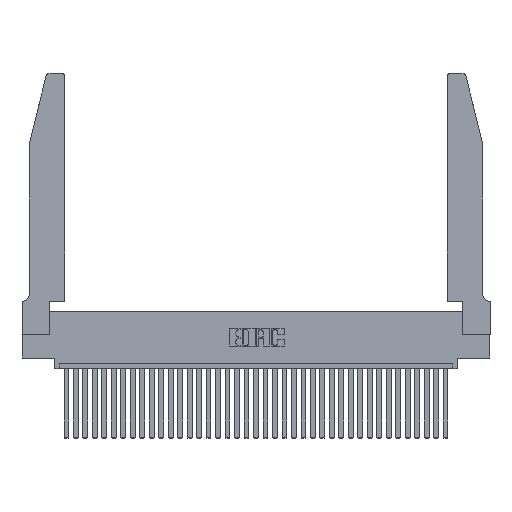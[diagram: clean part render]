
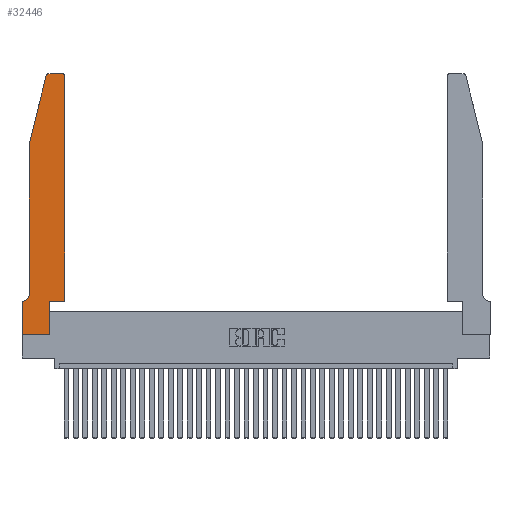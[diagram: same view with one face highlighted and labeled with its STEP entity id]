
A CAD part, top view. The second image highlights one B-rep face of the part: STEP entity #32446.
In plain terms, the highlighted planar face has unit normal (0, 0, 1).
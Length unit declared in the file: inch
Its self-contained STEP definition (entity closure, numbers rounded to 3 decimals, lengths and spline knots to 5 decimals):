
#397 = LINE ( 'NONE', #29421, #32304 ) ;
#413 = EDGE_CURVE ( 'NONE', #1160, #28381, #22873, .T. ) ;
#485 = VERTEX_POINT ( 'NONE', #21021 ) ;
#1160 = VERTEX_POINT ( 'NONE', #7438 ) ;
#1201 = DIRECTION ( 'NONE',  ( -1., 0., 0. ) ) ;
#1212 = DIRECTION ( 'NONE',  ( 1., 0., 0. ) ) ;
#1455 = VERTEX_POINT ( 'NONE', #33067 ) ;
#1555 = VERTEX_POINT ( 'NONE', #28013 ) ;
#2193 = CARTESIAN_POINT ( 'NONE',  ( 0.4505, 0.35, 0.37 ) ) ;
#2352 = DIRECTION ( 'NONE',  ( 0., 0., -1. ) ) ;
#2393 = EDGE_CURVE ( 'NONE', #11491, #25943, #9629, .T. ) ;
#2510 = CARTESIAN_POINT ( 'NONE',  ( 0.4505, 2.72, 0.37 ) ) ;
#3300 = EDGE_CURVE ( 'NONE', #22929, #11491, #6942, .T. ) ;
#3732 = CIRCLE ( 'NONE', #22625, 0.07 ) ;
#4644 = ORIENTED_EDGE ( 'NONE', *, *, #28030, .T. ) ;
#4886 = VECTOR ( 'NONE', #10353, 39.37008 ) ;
#5698 = VECTOR ( 'NONE', #12716, 39.37008 ) ;
#6319 = CARTESIAN_POINT ( 'NONE',  ( 0.4505, 0.35, 0.37 ) ) ;
#6451 = CARTESIAN_POINT ( 'NONE',  ( 0., 0.35, 0.37 ) ) ;
#6468 = ORIENTED_EDGE ( 'NONE', *, *, #8526, .T. ) ;
#6473 = ORIENTED_EDGE ( 'NONE', *, *, #2393, .T. ) ;
#6740 = EDGE_CURVE ( 'NONE', #22603, #1455, #11949, .T. ) ;
#6942 = LINE ( 'NONE', #7710, #12152 ) ;
#7042 = AXIS2_PLACEMENT_3D ( 'NONE', #28745, #23418, #1212 ) ;
#7438 = CARTESIAN_POINT ( 'NONE',  ( 0.4205, 2.75, 0.37 ) ) ;
#7710 = CARTESIAN_POINT ( 'NONE',  ( 0., 0., 0.37 ) ) ;
#8526 = EDGE_CURVE ( 'NONE', #14912, #1160, #12629, .T. ) ;
#9610 = ORIENTED_EDGE ( 'NONE', *, *, #413, .T. ) ;
#9629 = LINE ( 'NONE', #23744, #4886 ) ;
#10130 = CARTESIAN_POINT ( 'NONE',  ( 0.4505, 0.35, 0.37 ) ) ;
#10353 = DIRECTION ( 'NONE',  ( 0., 1., 0. ) ) ;
#11221 = DIRECTION ( 'NONE',  ( 1., 0., 0. ) ) ;
#11491 = VERTEX_POINT ( 'NONE', #14088 ) ;
#11625 = ORIENTED_EDGE ( 'NONE', *, *, #15113, .T. ) ;
#11651 = ORIENTED_EDGE ( 'NONE', *, *, #35454, .T. ) ;
#11795 = CARTESIAN_POINT ( 'NONE',  ( 0.284, 2.75, 0.37 ) ) ;
#11949 = LINE ( 'NONE', #20639, #27901 ) ;
#12152 = VECTOR ( 'NONE', #11221, 39.37008 ) ;
#12507 = VERTEX_POINT ( 'NONE', #6319 ) ;
#12611 = CARTESIAN_POINT ( 'NONE',  ( 0.0755, 2., 0.37 ) ) ;
#12629 = CIRCLE ( 'NONE', #19109, 0.03 ) ;
#12716 = DIRECTION ( 'NONE',  ( 0., -1., 0. ) ) ;
#13688 = VECTOR ( 'NONE', #29699, 39.37008 ) ;
#14088 = CARTESIAN_POINT ( 'NONE',  ( 0.2865, 0., 0.37 ) ) ;
#14380 = CARTESIAN_POINT ( 'NONE',  ( 0.2865, 0.35, 0.37 ) ) ;
#14547 = EDGE_LOOP ( 'NONE', ( #9610, #11651, #4644, #11625, #32239, #17628, #23482, #23383, #6473, #29335, #28878, #6468 ) ) ;
#14912 = VERTEX_POINT ( 'NONE', #2510 ) ;
#15113 = EDGE_CURVE ( 'NONE', #25020, #485, #27736, .T. ) ;
#15902 = DIRECTION ( 'NONE',  ( -0.239, -0.971, 0. ) ) ;
#17103 = CARTESIAN_POINT ( 'NONE',  ( 0.4205, 2.72, 0.37 ) ) ;
#17628 = ORIENTED_EDGE ( 'NONE', *, *, #6740, .T. ) ;
#18680 = DIRECTION ( 'NONE',  ( -1., 0., 0. ) ) ;
#19109 = AXIS2_PLACEMENT_3D ( 'NONE', #17103, #33848, #20126 ) ;
#19798 = EDGE_CURVE ( 'NONE', #1455, #22929, #27839, .T. ) ;
#20126 = DIRECTION ( 'NONE',  ( 1., 0., 0. ) ) ;
#20322 = DIRECTION ( 'NONE',  ( 1., 0., 0. ) ) ;
#20381 = CARTESIAN_POINT ( 'NONE',  ( 0.0755, 2., 0.37 ) ) ;
#20639 = CARTESIAN_POINT ( 'NONE',  ( 0.0755, 0.35, 0.37 ) ) ;
#20658 = CIRCLE ( 'NONE', #7042, 0.03 ) ;
#21021 = CARTESIAN_POINT ( 'NONE',  ( 0.0755, 0.42, 0.37 ) ) ;
#21270 = DIRECTION ( 'NONE',  ( -1., 0., 0. ) ) ;
#21317 = AXIS2_PLACEMENT_3D ( 'NONE', #6451, #25533, #20322 ) ;
#22603 = VERTEX_POINT ( 'NONE', #25861 ) ;
#22625 = AXIS2_PLACEMENT_3D ( 'NONE', #29740, #2352, #18680 ) ;
#22655 = CARTESIAN_POINT ( 'NONE',  ( 0., 0., 0.37 ) ) ;
#22873 = LINE ( 'NONE', #23821, #33674 ) ;
#22929 = VERTEX_POINT ( 'NONE', #22655 ) ;
#23383 = ORIENTED_EDGE ( 'NONE', *, *, #3300, .T. ) ;
#23418 = DIRECTION ( 'NONE',  ( 0., 0., 1. ) ) ;
#23482 = ORIENTED_EDGE ( 'NONE', *, *, #19798, .T. ) ;
#23744 = CARTESIAN_POINT ( 'NONE',  ( 0.2865, 0.35, 0.37 ) ) ;
#23821 = CARTESIAN_POINT ( 'NONE',  ( 0.2605, 2.75, 0.37 ) ) ;
#24839 = VECTOR ( 'NONE', #28596, 39.37008 ) ;
#25020 = VERTEX_POINT ( 'NONE', #20381 ) ;
#25533 = DIRECTION ( 'NONE',  ( 0., 0., 1. ) ) ;
#25861 = CARTESIAN_POINT ( 'NONE',  ( 0.0055, 0.35, 0.37 ) ) ;
#25943 = VERTEX_POINT ( 'NONE', #14380 ) ;
#27736 = LINE ( 'NONE', #12611, #5698 ) ;
#27839 = LINE ( 'NONE', #33878, #24839 ) ;
#27901 = VECTOR ( 'NONE', #1201, 39.37008 ) ;
#28013 = CARTESIAN_POINT ( 'NONE',  ( 0.25487, 2.72718, 0.37 ) ) ;
#28030 = EDGE_CURVE ( 'NONE', #1555, #25020, #397, .T. ) ;
#28381 = VERTEX_POINT ( 'NONE', #11795 ) ;
#28596 = DIRECTION ( 'NONE',  ( 0., -1., 0. ) ) ;
#28745 = CARTESIAN_POINT ( 'NONE',  ( 0.284, 2.72, 0.37 ) ) ;
#28878 = ORIENTED_EDGE ( 'NONE', *, *, #29696, .T. ) ;
#29184 = EDGE_CURVE ( 'NONE', #485, #22603, #3732, .T. ) ;
#29309 = DIRECTION ( 'NONE',  ( 1., 0., 0. ) ) ;
#29335 = ORIENTED_EDGE ( 'NONE', *, *, #32864, .T. ) ;
#29421 = CARTESIAN_POINT ( 'NONE',  ( 0.0755, 2., 0.37 ) ) ;
#29696 = EDGE_CURVE ( 'NONE', #12507, #14912, #34330, .T. ) ;
#29699 = DIRECTION ( 'NONE',  ( 0., 1., 0. ) ) ;
#29740 = CARTESIAN_POINT ( 'NONE',  ( 0.0055, 0.42, 0.37 ) ) ;
#31055 = LINE ( 'NONE', #10130, #32772 ) ;
#31263 = PLANE ( 'NONE',  #21317 ) ;
#32239 = ORIENTED_EDGE ( 'NONE', *, *, #29184, .T. ) ;
#32304 = VECTOR ( 'NONE', #15902, 39.37008 ) ;
#32446 = ADVANCED_FACE ( 'NONE', ( #34546 ), #31263, .T. ) ;
#32772 = VECTOR ( 'NONE', #29309, 39.37008 ) ;
#32864 = EDGE_CURVE ( 'NONE', #25943, #12507, #31055, .T. ) ;
#33067 = CARTESIAN_POINT ( 'NONE',  ( 0., 0.35, 0.37 ) ) ;
#33674 = VECTOR ( 'NONE', #21270, 39.37008 ) ;
#33848 = DIRECTION ( 'NONE',  ( 0., 0., 1. ) ) ;
#33878 = CARTESIAN_POINT ( 'NONE',  ( 0., 0., 0.37 ) ) ;
#34330 = LINE ( 'NONE', #2193, #13688 ) ;
#34546 = FACE_OUTER_BOUND ( 'NONE', #14547, .T. ) ;
#35454 = EDGE_CURVE ( 'NONE', #28381, #1555, #20658, .T. ) ;
